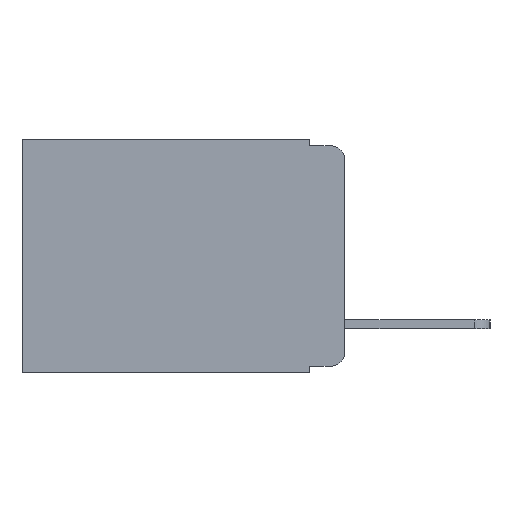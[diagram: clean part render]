
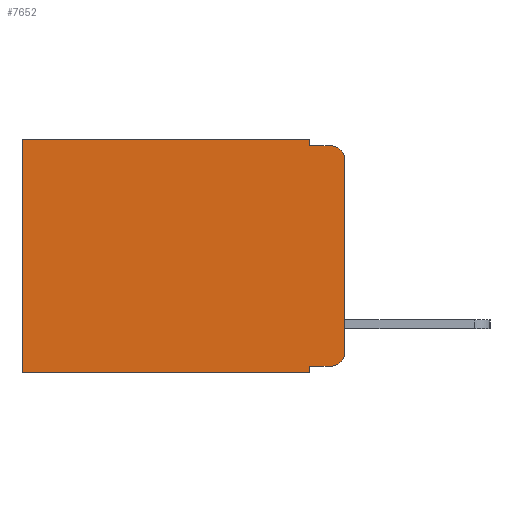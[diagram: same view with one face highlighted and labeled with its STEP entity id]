
A CAD part, left-side view. The second image highlights one B-rep face of the part: STEP entity #7652.
In plain terms, the highlighted planar face has unit normal (-1, 0, 0).
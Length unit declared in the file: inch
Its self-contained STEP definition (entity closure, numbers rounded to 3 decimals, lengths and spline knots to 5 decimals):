
#547 = CARTESIAN_POINT ( 'NONE',  ( 0.298, 0.473, 0. ) ) ;
#731 = LINE ( 'NONE', #547, #14758 ) ;
#1002 = EDGE_CURVE ( 'NONE', #1646, #17102, #17540, .T. ) ;
#1646 = VERTEX_POINT ( 'NONE', #18867 ) ;
#1695 = ORIENTED_EDGE ( 'NONE', *, *, #13485, .T. ) ;
#1873 = VECTOR ( 'NONE', #18629, 39.37008 ) ;
#2392 = AXIS2_PLACEMENT_3D ( 'NONE', #13041, #9285, #22403 ) ;
#2518 = CARTESIAN_POINT ( 'NONE',  ( 0.298, 0.051, 0. ) ) ;
#2531 = DIRECTION ( 'NONE',  ( 0., 0., -1. ) ) ;
#2545 = DIRECTION ( 'NONE',  ( 0., -1., 0. ) ) ;
#2553 = VERTEX_POINT ( 'NONE', #19212 ) ;
#2941 = CARTESIAN_POINT ( 'NONE',  ( 0.298, 0.051, -0.333 ) ) ;
#2942 = ORIENTED_EDGE ( 'NONE', *, *, #10343, .T. ) ;
#3087 = DIRECTION ( 'NONE',  ( 0., 1., 0. ) ) ;
#3334 = ORIENTED_EDGE ( 'NONE', *, *, #1002, .F. ) ;
#3548 = CARTESIAN_POINT ( 'NONE',  ( 0.298, 0., -0.313 ) ) ;
#4832 = ORIENTED_EDGE ( 'NONE', *, *, #18511, .T. ) ;
#4987 = ORIENTED_EDGE ( 'NONE', *, *, #20993, .F. ) ;
#5242 = CIRCLE ( 'NONE', #9088, 0.02 ) ;
#5495 = CARTESIAN_POINT ( 'NONE',  ( 0.298, 0., 0. ) ) ;
#5617 = AXIS2_PLACEMENT_3D ( 'NONE', #18496, #7184, #20360 ) ;
#5756 = CARTESIAN_POINT ( 'NONE',  ( 0.298, 0.051, 0. ) ) ;
#6196 = ORIENTED_EDGE ( 'NONE', *, *, #15989, .F. ) ;
#6271 = DIRECTION ( 'NONE',  ( 0., 0., -1. ) ) ;
#6721 = CARTESIAN_POINT ( 'NONE',  ( 0.298, 0.02, -0.333 ) ) ;
#6766 = DIRECTION ( 'NONE',  ( -1., 0., 0. ) ) ;
#6820 = VERTEX_POINT ( 'NONE', #2941 ) ;
#6877 = LINE ( 'NONE', #13937, #21287 ) ;
#6891 = VECTOR ( 'NONE', #15015, 39.37008 ) ;
#7184 = DIRECTION ( 'NONE',  ( -1., 0., 0. ) ) ;
#7206 = ORIENTED_EDGE ( 'NONE', *, *, #8396, .T. ) ;
#7528 = FACE_OUTER_BOUND ( 'NONE', #24171, .T. ) ;
#7652 = ADVANCED_FACE ( 'NONE', ( #7528 ), #20556, .F. ) ;
#8396 = EDGE_CURVE ( 'NONE', #15511, #18092, #5242, .T. ) ;
#8587 = ORIENTED_EDGE ( 'NONE', *, *, #14747, .F. ) ;
#8687 = DIRECTION ( 'NONE',  ( 0., -1., 0. ) ) ;
#9088 = AXIS2_PLACEMENT_3D ( 'NONE', #18083, #6766, #19969 ) ;
#9285 = DIRECTION ( 'NONE',  ( 1., 0., 0. ) ) ;
#9664 = EDGE_CURVE ( 'NONE', #6820, #15511, #15826, .T. ) ;
#10343 = EDGE_CURVE ( 'NONE', #20144, #2553, #21618, .T. ) ;
#10491 = VECTOR ( 'NONE', #3087, 39.37008 ) ;
#11283 = ORIENTED_EDGE ( 'NONE', *, *, #12225, .F. ) ;
#11868 = VERTEX_POINT ( 'NONE', #16020 ) ;
#12209 = ORIENTED_EDGE ( 'NONE', *, *, #9664, .T. ) ;
#12225 = EDGE_CURVE ( 'NONE', #6820, #1646, #18047, .T. ) ;
#12576 = CARTESIAN_POINT ( 'NONE',  ( 0.298, 0., 0. ) ) ;
#13041 = CARTESIAN_POINT ( 'NONE',  ( 0.298, 0., 0. ) ) ;
#13485 = EDGE_CURVE ( 'NONE', #2553, #17102, #731, .T. ) ;
#13906 = CARTESIAN_POINT ( 'NONE',  ( 0.298, 0.473, -0.343 ) ) ;
#13937 = CARTESIAN_POINT ( 'NONE',  ( 0.298, 0.051, -0.01 ) ) ;
#14167 = CIRCLE ( 'NONE', #5617, 0.02 ) ;
#14433 = VERTEX_POINT ( 'NONE', #16770 ) ;
#14747 = EDGE_CURVE ( 'NONE', #20144, #18166, #16394, .T. ) ;
#14758 = VECTOR ( 'NONE', #2531, 39.37008 ) ;
#15015 = DIRECTION ( 'NONE',  ( 0., 1., 0. ) ) ;
#15511 = VERTEX_POINT ( 'NONE', #6721 ) ;
#15826 = LINE ( 'NONE', #19992, #16404 ) ;
#15989 = EDGE_CURVE ( 'NONE', #18166, #14433, #6877, .T. ) ;
#16020 = CARTESIAN_POINT ( 'NONE',  ( 0.298, 0., -0.03 ) ) ;
#16394 = LINE ( 'NONE', #2518, #20780 ) ;
#16404 = VECTOR ( 'NONE', #8687, 39.37008 ) ;
#16441 = LINE ( 'NONE', #5495, #1873 ) ;
#16770 = CARTESIAN_POINT ( 'NONE',  ( 0.298, 0.02, -0.01 ) ) ;
#17102 = VERTEX_POINT ( 'NONE', #13906 ) ;
#17540 = LINE ( 'NONE', #20951, #6891 ) ;
#17868 = CARTESIAN_POINT ( 'NONE',  ( 0.298, 0.051, 0. ) ) ;
#18047 = LINE ( 'NONE', #5756, #22383 ) ;
#18083 = CARTESIAN_POINT ( 'NONE',  ( 0.298, 0.02, -0.313 ) ) ;
#18092 = VERTEX_POINT ( 'NONE', #3548 ) ;
#18166 = VERTEX_POINT ( 'NONE', #24467 ) ;
#18496 = CARTESIAN_POINT ( 'NONE',  ( 0.298, 0.02, -0.03 ) ) ;
#18511 = EDGE_CURVE ( 'NONE', #11868, #14433, #14167, .T. ) ;
#18629 = DIRECTION ( 'NONE',  ( 0., 0., -1. ) ) ;
#18867 = CARTESIAN_POINT ( 'NONE',  ( 0.298, 0.051, -0.343 ) ) ;
#19212 = CARTESIAN_POINT ( 'NONE',  ( 0.298, 0.473, 0. ) ) ;
#19969 = DIRECTION ( 'NONE',  ( 0., 0., -1. ) ) ;
#19992 = CARTESIAN_POINT ( 'NONE',  ( 0.298, 0.051, -0.333 ) ) ;
#20144 = VERTEX_POINT ( 'NONE', #17868 ) ;
#20360 = DIRECTION ( 'NONE',  ( 0., 0., -1. ) ) ;
#20556 = PLANE ( 'NONE',  #2392 ) ;
#20780 = VECTOR ( 'NONE', #6271, 39.37008 ) ;
#20895 = DIRECTION ( 'NONE',  ( 0., 0., -1. ) ) ;
#20951 = CARTESIAN_POINT ( 'NONE',  ( 0.298, 0., -0.343 ) ) ;
#20993 = EDGE_CURVE ( 'NONE', #11868, #18092, #16441, .T. ) ;
#21287 = VECTOR ( 'NONE', #2545, 39.37008 ) ;
#21618 = LINE ( 'NONE', #12576, #10491 ) ;
#22383 = VECTOR ( 'NONE', #20895, 39.37008 ) ;
#22403 = DIRECTION ( 'NONE',  ( 0., 0., -1. ) ) ;
#24171 = EDGE_LOOP ( 'NONE', ( #4987, #4832, #6196, #8587, #2942, #1695, #3334, #11283, #12209, #7206 ) ) ;
#24467 = CARTESIAN_POINT ( 'NONE',  ( 0.298, 0.051, -0.01 ) ) ;
